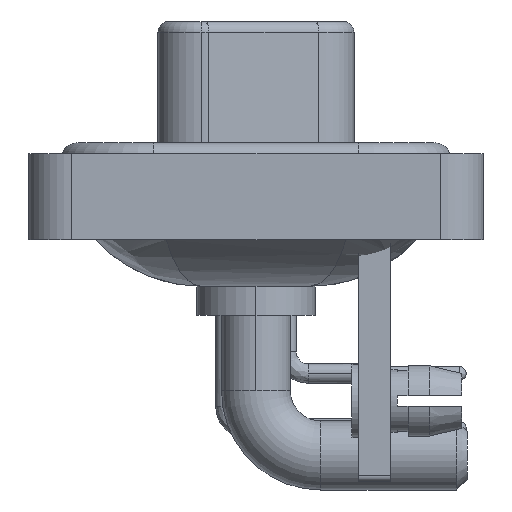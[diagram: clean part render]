
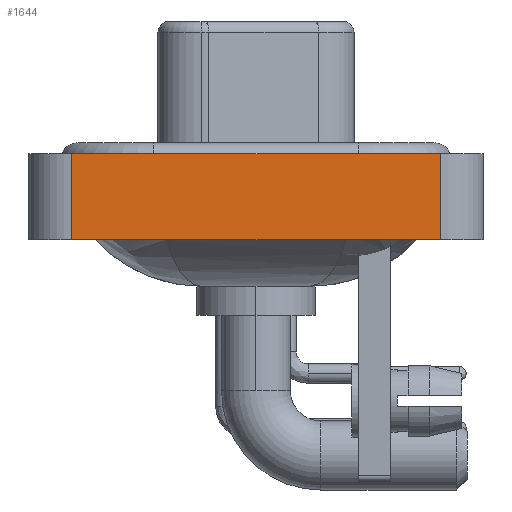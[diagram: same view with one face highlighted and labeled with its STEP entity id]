
A CAD part, left-side view. The second image highlights one B-rep face of the part: STEP entity #1644.
In plain terms, the highlighted planar face has unit normal (-1, 0, 0).
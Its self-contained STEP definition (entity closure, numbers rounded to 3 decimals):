
#314 = AXIS2_PLACEMENT_3D ( 'NONE', #892, #3311, #28780 ) ;
#405 = CARTESIAN_POINT ( 'NONE',  ( -7.35, -8.55, -3.6 ) ) ;
#892 = CARTESIAN_POINT ( 'NONE',  ( -7.35, -8.55, -3.6 ) ) ;
#1644 = ADVANCED_FACE ( 'NONE', ( #7650 ), #10498, .T. ) ;
#1756 = CARTESIAN_POINT ( 'NONE',  ( -7.35, 8.55, 0.4 ) ) ;
#3105 = LINE ( 'NONE', #22262, #8917 ) ;
#3311 = DIRECTION ( 'NONE',  ( -1., 0., 0. ) ) ;
#6195 = VERTEX_POINT ( 'NONE', #12564 ) ;
#7650 = FACE_OUTER_BOUND ( 'NONE', #8758, .T. ) ;
#8530 = VERTEX_POINT ( 'NONE', #405 ) ;
#8758 = EDGE_LOOP ( 'NONE', ( #14842, #24261, #27404, #13564 ) ) ;
#8886 = DIRECTION ( 'NONE',  ( 0., 0., 1. ) ) ;
#8917 = VECTOR ( 'NONE', #20009, 1000. ) ;
#9041 = CARTESIAN_POINT ( 'NONE',  ( -7.35, 8.55, -3.6 ) ) ;
#10498 = PLANE ( 'NONE',  #314 ) ;
#10550 = VECTOR ( 'NONE', #26970, 1000. ) ;
#11006 = LINE ( 'NONE', #20149, #14618 ) ;
#12564 = CARTESIAN_POINT ( 'NONE',  ( -7.35, -8.55, 0.4 ) ) ;
#13522 = CARTESIAN_POINT ( 'NONE',  ( -7.35, -8.55, -3.6 ) ) ;
#13564 = ORIENTED_EDGE ( 'NONE', *, *, #18306, .T. ) ;
#14389 = CARTESIAN_POINT ( 'NONE',  ( -7.35, 8.55, -3.6 ) ) ;
#14618 = VECTOR ( 'NONE', #29287, 1000. ) ;
#14842 = ORIENTED_EDGE ( 'NONE', *, *, #25935, .T. ) ;
#17729 = VECTOR ( 'NONE', #8886, 1000. ) ;
#18156 = LINE ( 'NONE', #13522, #10550 ) ;
#18306 = EDGE_CURVE ( 'NONE', #26079, #8530, #11006, .T. ) ;
#19365 = EDGE_CURVE ( 'NONE', #25246, #6195, #3105, .T. ) ;
#20009 = DIRECTION ( 'NONE',  ( 0., -1., 0. ) ) ;
#20149 = CARTESIAN_POINT ( 'NONE',  ( -7.35, -8.55, -3.6 ) ) ;
#22262 = CARTESIAN_POINT ( 'NONE',  ( -7.35, -8.55, 0.4 ) ) ;
#24261 = ORIENTED_EDGE ( 'NONE', *, *, #19365, .F. ) ;
#25209 = LINE ( 'NONE', #9041, #17729 ) ;
#25246 = VERTEX_POINT ( 'NONE', #1756 ) ;
#25705 = EDGE_CURVE ( 'NONE', #26079, #25246, #25209, .T. ) ;
#25935 = EDGE_CURVE ( 'NONE', #8530, #6195, #18156, .T. ) ;
#26079 = VERTEX_POINT ( 'NONE', #14389 ) ;
#26970 = DIRECTION ( 'NONE',  ( 0., 0., 1. ) ) ;
#27404 = ORIENTED_EDGE ( 'NONE', *, *, #25705, .F. ) ;
#28780 = DIRECTION ( 'NONE',  ( 0., 0., 1. ) ) ;
#29287 = DIRECTION ( 'NONE',  ( 0., -1., 0. ) ) ;
